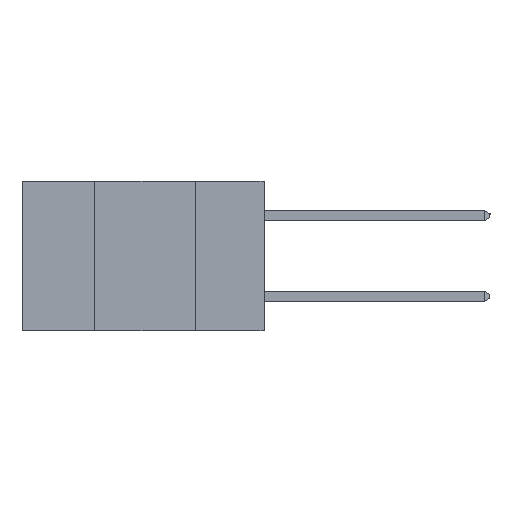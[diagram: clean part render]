
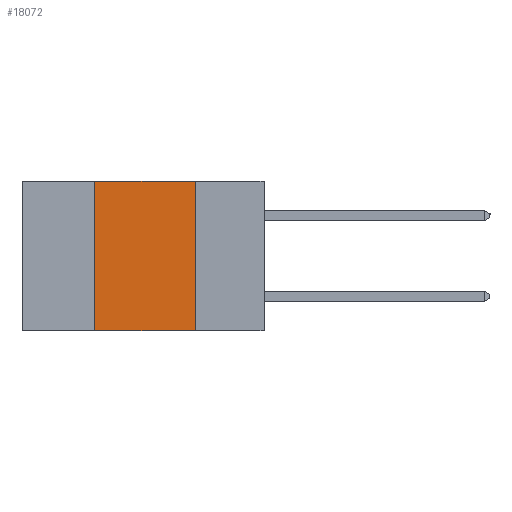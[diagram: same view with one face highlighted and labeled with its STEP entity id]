
A CAD part, left-side view. The second image highlights one B-rep face of the part: STEP entity #18072.
In plain terms, the highlighted planar face has unit normal (-1, 0, 0).
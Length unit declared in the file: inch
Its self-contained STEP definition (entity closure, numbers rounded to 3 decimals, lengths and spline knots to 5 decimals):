
#500 = LINE ( 'NONE', #10402, #13414 ) ;
#807 = CARTESIAN_POINT ( 'NONE',  ( 0., 0.6, 0. ) ) ;
#865 = DIRECTION ( 'NONE',  ( 0., 0., 1. ) ) ;
#2100 = EDGE_CURVE ( 'NONE', #3701, #19950, #500, .T. ) ;
#2221 = VERTEX_POINT ( 'NONE', #11842 ) ;
#2470 = AXIS2_PLACEMENT_3D ( 'NONE', #807, #21279, #6183 ) ;
#2551 = PLANE ( 'NONE',  #2470 ) ;
#2763 = LINE ( 'NONE', #14026, #3376 ) ;
#3376 = VECTOR ( 'NONE', #9494, 39.37008 ) ;
#3701 = VERTEX_POINT ( 'NONE', #18312 ) ;
#4646 = CARTESIAN_POINT ( 'NONE',  ( 0., 0.17, -0.37 ) ) ;
#6183 = DIRECTION ( 'NONE',  ( 0., 0., -1. ) ) ;
#6699 = ORIENTED_EDGE ( 'NONE', *, *, #7191, .T. ) ;
#7191 = EDGE_CURVE ( 'NONE', #2221, #19950, #2763, .T. ) ;
#7859 = FACE_OUTER_BOUND ( 'NONE', #9000, .T. ) ;
#9000 = EDGE_LOOP ( 'NONE', ( #17831, #14831, #11496, #6699 ) ) ;
#9462 = VECTOR ( 'NONE', #865, 39.37008 ) ;
#9494 = DIRECTION ( 'NONE',  ( 0., -1., 0. ) ) ;
#9958 = EDGE_CURVE ( 'NONE', #13278, #3701, #17604, .T. ) ;
#10402 = CARTESIAN_POINT ( 'NONE',  ( 0., 0.17, -0.37 ) ) ;
#11496 = ORIENTED_EDGE ( 'NONE', *, *, #17000, .F. ) ;
#11842 = CARTESIAN_POINT ( 'NONE',  ( 0., 0.42, -0.37 ) ) ;
#13094 = VECTOR ( 'NONE', #21153, 39.37008 ) ;
#13278 = VERTEX_POINT ( 'NONE', #18257 ) ;
#13414 = VECTOR ( 'NONE', #15445, 39.37008 ) ;
#14026 = CARTESIAN_POINT ( 'NONE',  ( 0., 0.6, -0.37 ) ) ;
#14831 = ORIENTED_EDGE ( 'NONE', *, *, #9958, .F. ) ;
#15445 = DIRECTION ( 'NONE',  ( 0., 0., -1. ) ) ;
#15908 = CARTESIAN_POINT ( 'NONE',  ( 0., 0.42, -0.37 ) ) ;
#17000 = EDGE_CURVE ( 'NONE', #2221, #13278, #20747, .T. ) ;
#17604 = LINE ( 'NONE', #19489, #13094 ) ;
#17831 = ORIENTED_EDGE ( 'NONE', *, *, #2100, .F. ) ;
#18072 = ADVANCED_FACE ( 'NONE', ( #7859 ), #2551, .F. ) ;
#18257 = CARTESIAN_POINT ( 'NONE',  ( 0., 0.42, 0. ) ) ;
#18312 = CARTESIAN_POINT ( 'NONE',  ( 0., 0.17, 0. ) ) ;
#19489 = CARTESIAN_POINT ( 'NONE',  ( 0., 0.6, 0. ) ) ;
#19950 = VERTEX_POINT ( 'NONE', #4646 ) ;
#20747 = LINE ( 'NONE', #15908, #9462 ) ;
#21153 = DIRECTION ( 'NONE',  ( 0., -1., 0. ) ) ;
#21279 = DIRECTION ( 'NONE',  ( 1., 0., 0. ) ) ;
